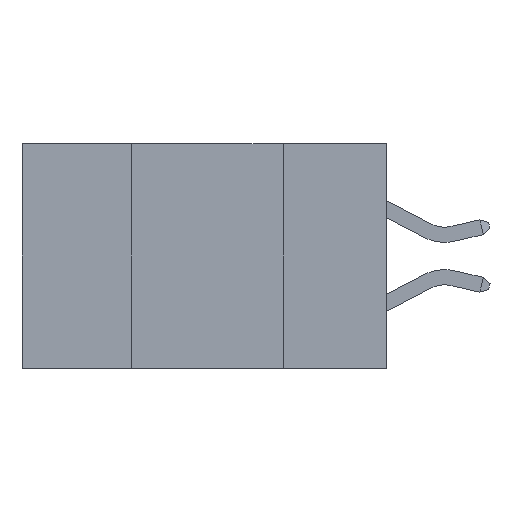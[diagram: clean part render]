
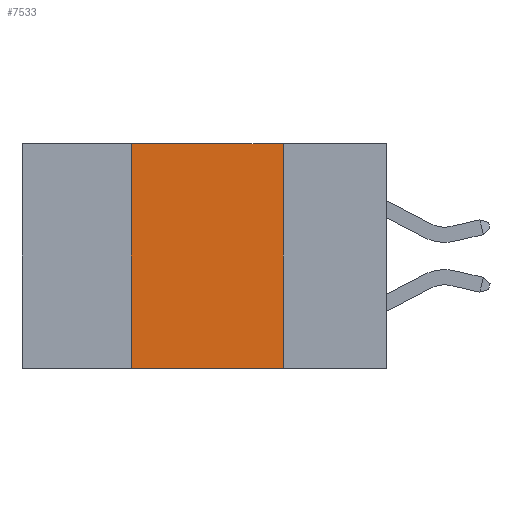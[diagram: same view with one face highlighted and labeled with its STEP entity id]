
A CAD part, left-side view. The second image highlights one B-rep face of the part: STEP entity #7533.
In plain terms, the highlighted planar face has unit normal (-1, 0, 0).
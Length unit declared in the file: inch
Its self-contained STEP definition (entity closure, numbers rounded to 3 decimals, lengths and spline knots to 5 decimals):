
#716 = ORIENTED_EDGE ( 'NONE', *, *, #11138, .F. ) ;
#1198 = VERTEX_POINT ( 'NONE', #11827 ) ;
#1313 = CARTESIAN_POINT ( 'NONE',  ( 0., 0.17, 0. ) ) ;
#1398 = VERTEX_POINT ( 'NONE', #15591 ) ;
#1676 = CARTESIAN_POINT ( 'NONE',  ( 0., 0.6, -0.37 ) ) ;
#1977 = CARTESIAN_POINT ( 'NONE',  ( 0., 0.6, 0. ) ) ;
#2677 = DIRECTION ( 'NONE',  ( 0., 0., -1. ) ) ;
#2797 = VECTOR ( 'NONE', #7261, 39.37008 ) ;
#3202 = LINE ( 'NONE', #1977, #2797 ) ;
#3495 = CARTESIAN_POINT ( 'NONE',  ( 0., 0.42, 0. ) ) ;
#3923 = LINE ( 'NONE', #1313, #14001 ) ;
#4244 = DIRECTION ( 'NONE',  ( 0., -1., 0. ) ) ;
#4389 = ORIENTED_EDGE ( 'NONE', *, *, #9334, .F. ) ;
#4625 = CARTESIAN_POINT ( 'NONE',  ( 0., 0.6, 0. ) ) ;
#4685 = DIRECTION ( 'NONE',  ( 0., 0., -1. ) ) ;
#5110 = AXIS2_PLACEMENT_3D ( 'NONE', #4625, #16722, #4685 ) ;
#7261 = DIRECTION ( 'NONE',  ( 0., -1., 0. ) ) ;
#7533 = ADVANCED_FACE ( 'NONE', ( #13953 ), #11441, .F. ) ;
#7743 = EDGE_CURVE ( 'NONE', #7927, #1398, #7822, .T. ) ;
#7822 = LINE ( 'NONE', #3495, #16487 ) ;
#7927 = VERTEX_POINT ( 'NONE', #8274 ) ;
#7983 = VECTOR ( 'NONE', #4244, 39.37008 ) ;
#8274 = CARTESIAN_POINT ( 'NONE',  ( 0., 0.42, -0.37 ) ) ;
#9334 = EDGE_CURVE ( 'NONE', #1398, #1198, #3202, .T. ) ;
#9645 = EDGE_CURVE ( 'NONE', #7927, #15224, #11574, .T. ) ;
#10232 = DIRECTION ( 'NONE',  ( 0., 0., 1. ) ) ;
#10652 = CARTESIAN_POINT ( 'NONE',  ( 0., 0.17, -0.37 ) ) ;
#10876 = ORIENTED_EDGE ( 'NONE', *, *, #7743, .F. ) ;
#11138 = EDGE_CURVE ( 'NONE', #1198, #15224, #3923, .T. ) ;
#11441 = PLANE ( 'NONE',  #5110 ) ;
#11574 = LINE ( 'NONE', #1676, #7983 ) ;
#11827 = CARTESIAN_POINT ( 'NONE',  ( 0., 0.17, 0. ) ) ;
#12613 = ORIENTED_EDGE ( 'NONE', *, *, #9645, .T. ) ;
#13447 = EDGE_LOOP ( 'NONE', ( #716, #4389, #10876, #12613 ) ) ;
#13953 = FACE_OUTER_BOUND ( 'NONE', #13447, .T. ) ;
#14001 = VECTOR ( 'NONE', #2677, 39.37008 ) ;
#15224 = VERTEX_POINT ( 'NONE', #10652 ) ;
#15591 = CARTESIAN_POINT ( 'NONE',  ( 0., 0.42, 0. ) ) ;
#16487 = VECTOR ( 'NONE', #10232, 39.37008 ) ;
#16722 = DIRECTION ( 'NONE',  ( 1., 0., 0. ) ) ;
